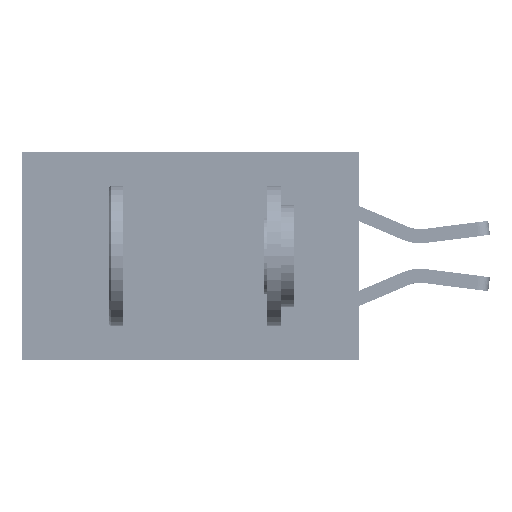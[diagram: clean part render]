
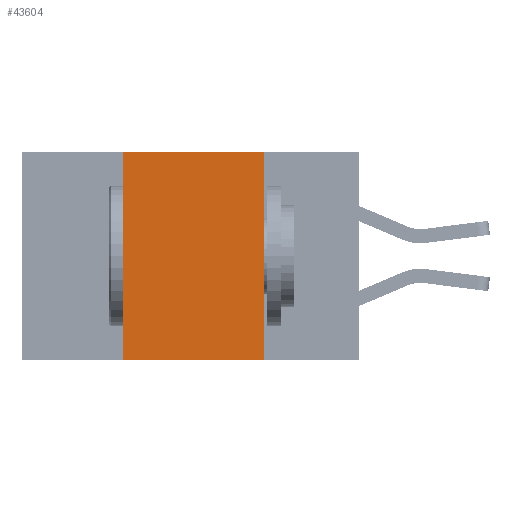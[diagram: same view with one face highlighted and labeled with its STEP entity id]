
A CAD part, left-side view. The second image highlights one B-rep face of the part: STEP entity #43604.
In plain terms, the highlighted planar face has unit normal (-1, 0, 0).
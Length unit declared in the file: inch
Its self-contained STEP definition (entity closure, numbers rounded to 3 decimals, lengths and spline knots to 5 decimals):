
#1652 = AXIS2_PLACEMENT_3D ( 'NONE', #6109, #30478, #9626 ) ;
#2005 = VECTOR ( 'NONE', #12423, 39.37008 ) ;
#4701 = ORIENTED_EDGE ( 'NONE', *, *, #6933, .F. ) ;
#5234 = EDGE_CURVE ( 'NONE', #44458, #22343, #5891, .T. ) ;
#5891 = LINE ( 'NONE', #41356, #31482 ) ;
#6109 = CARTESIAN_POINT ( 'NONE',  ( 0., 0.6, 0. ) ) ;
#6933 = EDGE_CURVE ( 'NONE', #13407, #17176, #17749, .T. ) ;
#9626 = DIRECTION ( 'NONE',  ( 0., 0., -1. ) ) ;
#12423 = DIRECTION ( 'NONE',  ( 0., 0., -1. ) ) ;
#12848 = EDGE_CURVE ( 'NONE', #44458, #13407, #40966, .T. ) ;
#13218 = VECTOR ( 'NONE', #24142, 39.37008 ) ;
#13407 = VERTEX_POINT ( 'NONE', #17145 ) ;
#16656 = VECTOR ( 'NONE', #40612, 39.37008 ) ;
#16812 = EDGE_LOOP ( 'NONE', ( #22160, #4701, #43908, #23814 ) ) ;
#16906 = CARTESIAN_POINT ( 'NONE',  ( 0., 0.17, -0.37 ) ) ;
#17145 = CARTESIAN_POINT ( 'NONE',  ( 0., 0.42, 0. ) ) ;
#17176 = VERTEX_POINT ( 'NONE', #29644 ) ;
#17749 = LINE ( 'NONE', #44081, #16656 ) ;
#18734 = FACE_OUTER_BOUND ( 'NONE', #16812, .T. ) ;
#20000 = PLANE ( 'NONE',  #1652 ) ;
#20666 = CARTESIAN_POINT ( 'NONE',  ( 0., 0.42, 0. ) ) ;
#22160 = ORIENTED_EDGE ( 'NONE', *, *, #39962, .F. ) ;
#22343 = VERTEX_POINT ( 'NONE', #16906 ) ;
#23814 = ORIENTED_EDGE ( 'NONE', *, *, #5234, .T. ) ;
#24142 = DIRECTION ( 'NONE',  ( 0., 0., 1. ) ) ;
#24631 = CARTESIAN_POINT ( 'NONE',  ( 0., 0.42, -0.37 ) ) ;
#28788 = LINE ( 'NONE', #40251, #2005 ) ;
#29644 = CARTESIAN_POINT ( 'NONE',  ( 0., 0.17, 0. ) ) ;
#30478 = DIRECTION ( 'NONE',  ( 1., 0., 0. ) ) ;
#31482 = VECTOR ( 'NONE', #34509, 39.37008 ) ;
#34509 = DIRECTION ( 'NONE',  ( 0., -1., 0. ) ) ;
#39962 = EDGE_CURVE ( 'NONE', #17176, #22343, #28788, .T. ) ;
#40251 = CARTESIAN_POINT ( 'NONE',  ( 0., 0.17, 0. ) ) ;
#40612 = DIRECTION ( 'NONE',  ( 0., -1., 0. ) ) ;
#40966 = LINE ( 'NONE', #20666, #13218 ) ;
#41356 = CARTESIAN_POINT ( 'NONE',  ( 0., 0.6, -0.37 ) ) ;
#43604 = ADVANCED_FACE ( 'NONE', ( #18734 ), #20000, .F. ) ;
#43908 = ORIENTED_EDGE ( 'NONE', *, *, #12848, .F. ) ;
#44081 = CARTESIAN_POINT ( 'NONE',  ( 0., 0.6, 0. ) ) ;
#44458 = VERTEX_POINT ( 'NONE', #24631 ) ;
